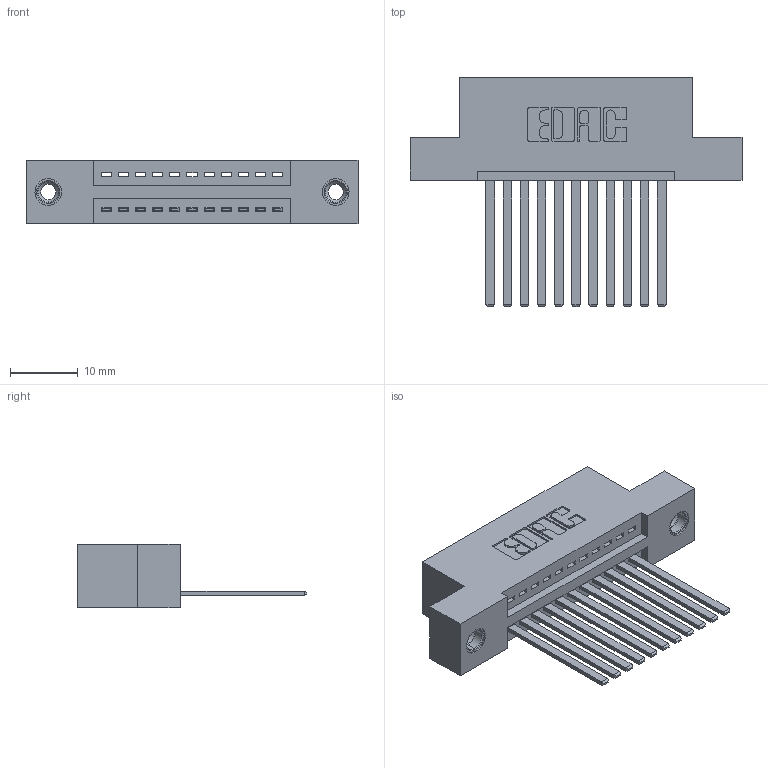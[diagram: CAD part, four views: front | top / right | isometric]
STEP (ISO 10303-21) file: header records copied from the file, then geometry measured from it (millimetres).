
FILE_DESCRIPTION (( 'STEP AP203' ), '1' );
FILE_NAME ('345-011-544-108.STEP', '2019-10-04T00:22:48', ( '' ), ( '' ), 'SwSTEP 2.0', 'SolidWorks 2016', '' );
FILE_SCHEMA (( 'CONFIG_CONTROL_DESIGN' ));
Length unit declared in the file: inch
Products named in the file (4): 345 Part_Flush Mounting Lugs - 0.156 Dia-TI; 345-292-001_345-293-144; 345-250-001_345-250-003-102; 345-011-544-108
Assembly tree (14 placements, depth 2):
  345-011-544-108
    345 Part_Flush Mounting Lugs - 0.156 Dia-TI
    345-292-001_345-293-144  x11
    345-250-001_345-250-003-102  x2
Bounding box: 49.15 x 33.96 x 9.4 mm (x, y, z)
Volume: 4535.2 mm3; surface area: 6007.1 mm2
Topology: 14 solids, 14 shells, 758 faces, 2215 edges, 1454 vertices
Faces by surface type: plane 508, cylinder 234, cone 12, torus 4
Entity records: 13454 total; most frequent: CARTESIAN_POINT 2312, ORIENTED_EDGE 2250, DIRECTION 2089, EDGE_CURVE 1125, LINE 933, VECTOR 933, VERTEX_POINT 744, AXIS2_PLACEMENT_3D 578
